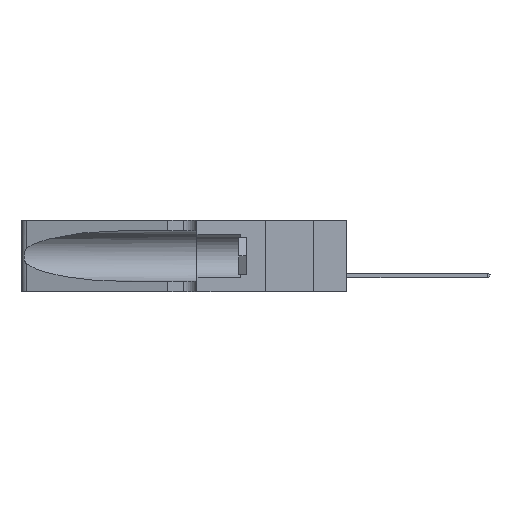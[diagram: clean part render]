
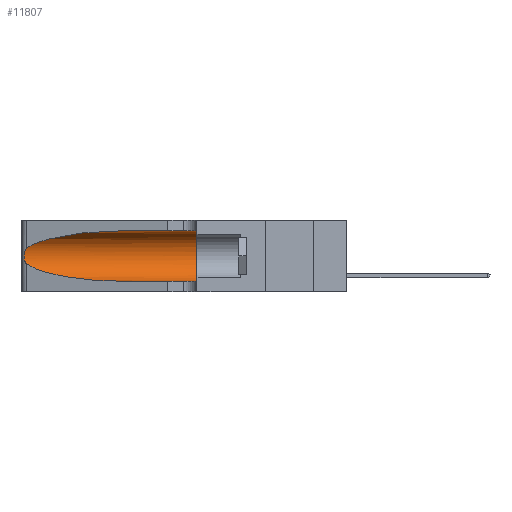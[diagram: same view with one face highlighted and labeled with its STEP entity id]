
A CAD part, left-side view. The second image highlights one B-rep face of the part: STEP entity #11807.
In plain terms, the highlighted cylindrical face has radius 3.308 mm (diameter 6.617 mm), a partial arc.
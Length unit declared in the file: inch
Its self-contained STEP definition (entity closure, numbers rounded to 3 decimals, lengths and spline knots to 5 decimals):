
#603 =( BOUNDED_CURVE ( )  B_SPLINE_CURVE ( 3, ( #43604, #40255, #51520, #47648 ),
 .UNSPECIFIED., .F., .F. ) 
 B_SPLINE_CURVE_WITH_KNOTS ( ( 4, 4 ),
 ( 3.44316, 4.71239 ),
 .UNSPECIFIED. ) 
 CURVE ( )  GEOMETRIC_REPRESENTATION_ITEM ( )  RATIONAL_B_SPLINE_CURVE ( ( 1., 0.87, 0.87, 1. ) ) 
 REPRESENTATION_ITEM ( '' )  );
#746 = CARTESIAN_POINT ( 'NONE',  ( 0.25487, 1.22718, 0.14631 ) ) ;
#1367 = CARTESIAN_POINT ( 'NONE',  ( 0.25854, 1.2359, 0.20912 ) ) ;
#1564 = CARTESIAN_POINT ( 'NONE',  ( 0.26075, 1.23896, 0.178 ) ) ;
#2586 = CARTESIAN_POINT ( 'NONE',  ( 0.1305, 1.61858, 0.31525 ) ) ;
#3380 = CYLINDRICAL_SURFACE ( 'NONE', #34083, 0.13025 ) ;
#4013 = FACE_OUTER_BOUND ( 'NONE', #41849, .T. ) ;
#4640 = EDGE_CURVE ( 'NONE', #32716, #10610, #14265, .T. ) ;
#5093 = CARTESIAN_POINT ( 'NONE',  ( 0.26018, 1.23835, 0.19895 ) ) ;
#5636 = CARTESIAN_POINT ( 'NONE',  ( 0.25856, 1.23593, 0.16098 ) ) ;
#6607 = CARTESIAN_POINT ( 'NONE',  ( 0.25487, 1.22718, 0.14631 ) ) ;
#8427 = ORIENTED_EDGE ( 'NONE', *, *, #17923, .T. ) ;
#8646 = EDGE_CURVE ( 'NONE', #32110, #30799, #22794, .T. ) ;
#8690 = EDGE_CURVE ( 'NONE', #39005, #10610, #24457, .T. ) ;
#8756 = DIRECTION ( 'NONE',  ( 0., -1., 0. ) ) ;
#8788 = CARTESIAN_POINT ( 'NONE',  ( 0.1305, 1.61858, 0.05475 ) ) ;
#9114 = CARTESIAN_POINT ( 'NONE',  ( 0.26075, 1.23896, 0.19203 ) ) ;
#10610 = VERTEX_POINT ( 'NONE', #38073 ) ;
#10893 = EDGE_CURVE ( 'NONE', #32110, #32716, #49770, .T. ) ;
#11807 = ADVANCED_FACE ( 'NONE', ( #4013 ), #3380, .F. ) ;
#14265 = CIRCLE ( 'NONE', #19560, 0.13025 ) ;
#14649 = CARTESIAN_POINT ( 'NONE',  ( 0.1305, 1.61858, 0.185 ) ) ;
#15045 = DIRECTION ( 'NONE',  ( 0., 1., 0. ) ) ;
#16484 = CARTESIAN_POINT ( 'NONE',  ( 0.25487, 1.22718, 0.22369 ) ) ;
#16612 = ORIENTED_EDGE ( 'NONE', *, *, #43515, .T. ) ;
#17923 = EDGE_CURVE ( 'NONE', #30799, #48840, #51617, .T. ) ;
#18449 = DIRECTION ( 'NONE',  ( 0., 0., -1. ) ) ;
#18712 = VECTOR ( 'NONE', #19184, 39.37008 ) ;
#19184 = DIRECTION ( 'NONE',  ( 0., -1., 0. ) ) ;
#19560 = AXIS2_PLACEMENT_3D ( 'NONE', #23025, #15045, #27104 ) ;
#19734 = CARTESIAN_POINT ( 'NONE',  ( 0.18966, 0.96281, 0.31525 ) ) ;
#22794 =( BOUNDED_CURVE ( )  B_SPLINE_CURVE ( 3, ( #30586, #19734, #35308, #43454 ),
 .UNSPECIFIED., .F., .F. ) 
 B_SPLINE_CURVE_WITH_KNOTS ( ( 4, 4 ),
 ( 1.5708, 2.84003 ),
 .UNSPECIFIED. ) 
 CURVE ( )  GEOMETRIC_REPRESENTATION_ITEM ( )  RATIONAL_B_SPLINE_CURVE ( ( 1., 0.87, 0.87, 1. ) ) 
 REPRESENTATION_ITEM ( '' )  );
#23025 = CARTESIAN_POINT ( 'NONE',  ( 0.1305, 0.35, 0.185 ) ) ;
#24457 = LINE ( 'NONE', #8788, #44950 ) ;
#24635 = CARTESIAN_POINT ( 'NONE',  ( 0.25555, 1.22994, 0.2215 ) ) ;
#24788 = CARTESIAN_POINT ( 'NONE',  ( 0.25787, 1.23484, 0.2124 ) ) ;
#25681 = CARTESIAN_POINT ( 'NONE',  ( 0.25789, 1.23486, 0.15765 ) ) ;
#26135 = ORIENTED_EDGE ( 'NONE', *, *, #8690, .T. ) ;
#26562 = CARTESIAN_POINT ( 'NONE',  ( 0.1305, 0.72297, 0.31525 ) ) ;
#27048 = DIRECTION ( 'NONE',  ( 0., -1., 0. ) ) ;
#27104 = DIRECTION ( 'NONE',  ( 0., 0., 1. ) ) ;
#30497 = CARTESIAN_POINT ( 'NONE',  ( 0.25639, 1.23186, 0.15144 ) ) ;
#30586 = CARTESIAN_POINT ( 'NONE',  ( 0.1305, 0.72297, 0.31525 ) ) ;
#30799 = VERTEX_POINT ( 'NONE', #44333 ) ;
#31726 = ORIENTED_EDGE ( 'NONE', *, *, #8646, .T. ) ;
#32110 = VERTEX_POINT ( 'NONE', #26562 ) ;
#32716 = VERTEX_POINT ( 'NONE', #34334 ) ;
#33363 = CARTESIAN_POINT ( 'NONE',  ( 0.26017, 1.23833, 0.17102 ) ) ;
#34067 = ORIENTED_EDGE ( 'NONE', *, *, #4640, .F. ) ;
#34083 = AXIS2_PLACEMENT_3D ( 'NONE', #14649, #27048, #18449 ) ;
#34334 = CARTESIAN_POINT ( 'NONE',  ( 0.1305, 0.35, 0.31525 ) ) ;
#35308 = CARTESIAN_POINT ( 'NONE',  ( 0.2373, 1.15595, 0.28018 ) ) ;
#36961 = ORIENTED_EDGE ( 'NONE', *, *, #10893, .F. ) ;
#38073 = CARTESIAN_POINT ( 'NONE',  ( 0.1305, 0.35, 0.05475 ) ) ;
#39005 = VERTEX_POINT ( 'NONE', #40654 ) ;
#40255 = CARTESIAN_POINT ( 'NONE',  ( 0.2373, 1.15595, 0.08982 ) ) ;
#40654 = CARTESIAN_POINT ( 'NONE',  ( 0.1305, 0.72297, 0.05475 ) ) ;
#41849 = EDGE_LOOP ( 'NONE', ( #31726, #8427, #16612, #26135, #34067, #36961 ) ) ;
#43454 = CARTESIAN_POINT ( 'NONE',  ( 0.25487, 1.22718, 0.22369 ) ) ;
#43515 = EDGE_CURVE ( 'NONE', #48840, #39005, #603, .T. ) ;
#43604 = CARTESIAN_POINT ( 'NONE',  ( 0.25487, 1.22718, 0.14631 ) ) ;
#44198 = CARTESIAN_POINT ( 'NONE',  ( 0.25639, 1.23184, 0.21858 ) ) ;
#44333 = CARTESIAN_POINT ( 'NONE',  ( 0.25487, 1.22718, 0.22369 ) ) ;
#44950 = VECTOR ( 'NONE', #8756, 39.37008 ) ;
#46123 = CARTESIAN_POINT ( 'NONE',  ( 0.25555, 1.22993, 0.14849 ) ) ;
#47648 = CARTESIAN_POINT ( 'NONE',  ( 0.1305, 0.72297, 0.05475 ) ) ;
#48840 = VERTEX_POINT ( 'NONE', #746 ) ;
#49770 = LINE ( 'NONE', #2586, #18712 ) ;
#51520 = CARTESIAN_POINT ( 'NONE',  ( 0.18966, 0.96281, 0.05475 ) ) ;
#51617 = B_SPLINE_CURVE_WITH_KNOTS ( 'NONE', 3,
 ( #16484, #24635, #44198, #24788, #1367, #5093, #9114, #1564, #33363, #5636, #25681, #30497, #46123, #6607 ),
 .UNSPECIFIED., .F., .F.,
 ( 4, 2, 2, 2, 2, 2, 4 ),
 ( 0., 0.00027, 0.00053, 0.00107, 0.0016, 0.00187, 0.00214 ),
 .UNSPECIFIED. ) ;
